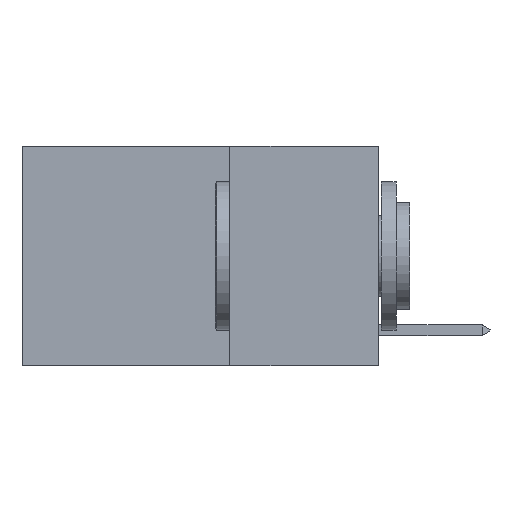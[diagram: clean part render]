
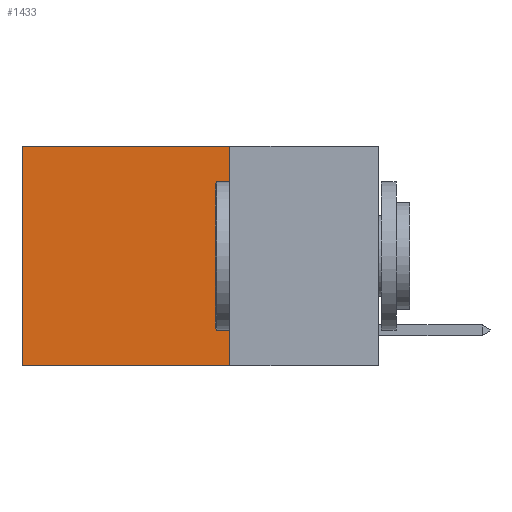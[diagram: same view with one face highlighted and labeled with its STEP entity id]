
A CAD part, left-side view. The second image highlights one B-rep face of the part: STEP entity #1433.
In plain terms, the highlighted planar face has unit normal (-1, 0, 0).
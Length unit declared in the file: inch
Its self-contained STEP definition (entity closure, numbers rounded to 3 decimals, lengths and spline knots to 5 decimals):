
#1143 = ORIENTED_EDGE ( 'NONE', *, *, #8174, .T. ) ;
#1222 = DIRECTION ( 'NONE',  ( 0., 0., -1. ) ) ;
#1305 = CARTESIAN_POINT ( 'NONE',  ( 0.2625, 0.25, 0. ) ) ;
#1397 = VECTOR ( 'NONE', #20695, 39.37008 ) ;
#1433 = ADVANCED_FACE ( 'NONE', ( #18281 ), #14409, .F. ) ;
#2740 = DIRECTION ( 'NONE',  ( 0., 0., -1. ) ) ;
#3274 = CARTESIAN_POINT ( 'NONE',  ( 0.2625, 0.25, 0. ) ) ;
#3685 = EDGE_LOOP ( 'NONE', ( #1143, #27812, #27977, #10308 ) ) ;
#4494 = AXIS2_PLACEMENT_3D ( 'NONE', #1305, #27043, #11986 ) ;
#4865 = LINE ( 'NONE', #26753, #8197 ) ;
#5469 = LINE ( 'NONE', #20771, #16366 ) ;
#6135 = EDGE_CURVE ( 'NONE', #18054, #24222, #27159, .T. ) ;
#6922 = EDGE_CURVE ( 'NONE', #18054, #19273, #5469, .T. ) ;
#8174 = EDGE_CURVE ( 'NONE', #24222, #15590, #4865, .T. ) ;
#8197 = VECTOR ( 'NONE', #2740, 39.37008 ) ;
#8703 = DIRECTION ( 'NONE',  ( 0., 1., 0. ) ) ;
#9697 = VECTOR ( 'NONE', #8703, 39.37008 ) ;
#10308 = ORIENTED_EDGE ( 'NONE', *, *, #6135, .T. ) ;
#11986 = DIRECTION ( 'NONE',  ( 0., 0., -1. ) ) ;
#12878 = CARTESIAN_POINT ( 'NONE',  ( 0.2625, 0.25, -0.37 ) ) ;
#14409 = PLANE ( 'NONE',  #4494 ) ;
#15034 = CARTESIAN_POINT ( 'NONE',  ( 0.2625, 0.25, 0. ) ) ;
#15294 = LINE ( 'NONE', #12878, #9697 ) ;
#15588 = EDGE_CURVE ( 'NONE', #19273, #15590, #15294, .T. ) ;
#15590 = VERTEX_POINT ( 'NONE', #26213 ) ;
#16366 = VECTOR ( 'NONE', #1222, 39.37008 ) ;
#18054 = VERTEX_POINT ( 'NONE', #15034 ) ;
#18281 = FACE_OUTER_BOUND ( 'NONE', #3685, .T. ) ;
#19273 = VERTEX_POINT ( 'NONE', #26105 ) ;
#20695 = DIRECTION ( 'NONE',  ( 0., 1., 0. ) ) ;
#20771 = CARTESIAN_POINT ( 'NONE',  ( 0.2625, 0.25, 0. ) ) ;
#21106 = CARTESIAN_POINT ( 'NONE',  ( 0.2625, 0.6, 0. ) ) ;
#24222 = VERTEX_POINT ( 'NONE', #21106 ) ;
#26105 = CARTESIAN_POINT ( 'NONE',  ( 0.2625, 0.25, -0.37 ) ) ;
#26213 = CARTESIAN_POINT ( 'NONE',  ( 0.2625, 0.6, -0.37 ) ) ;
#26753 = CARTESIAN_POINT ( 'NONE',  ( 0.2625, 0.6, 0. ) ) ;
#27043 = DIRECTION ( 'NONE',  ( 1., 0., 0. ) ) ;
#27159 = LINE ( 'NONE', #3274, #1397 ) ;
#27812 = ORIENTED_EDGE ( 'NONE', *, *, #15588, .F. ) ;
#27977 = ORIENTED_EDGE ( 'NONE', *, *, #6922, .F. ) ;
